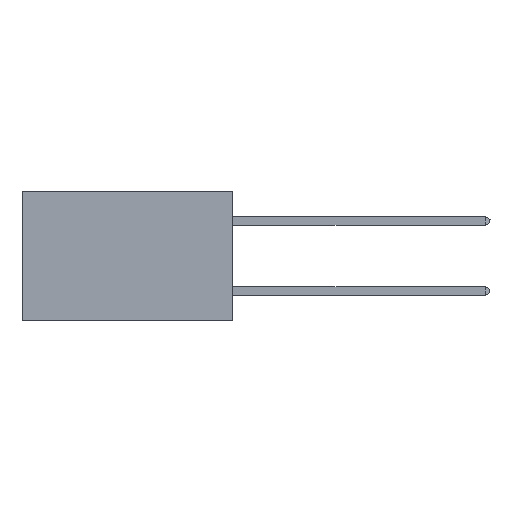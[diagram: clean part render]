
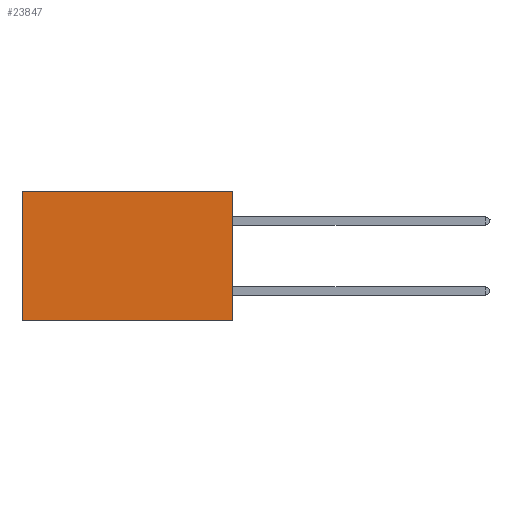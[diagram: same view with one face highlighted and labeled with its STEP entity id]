
A CAD part, left-side view. The second image highlights one B-rep face of the part: STEP entity #23847.
In plain terms, the highlighted planar face has unit normal (-1, 0, 0).
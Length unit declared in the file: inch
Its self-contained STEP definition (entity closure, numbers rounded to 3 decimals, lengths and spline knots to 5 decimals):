
#1172 = AXIS2_PLACEMENT_3D ( 'NONE', #16849, #28862, #4880 ) ;
#2089 = DIRECTION ( 'NONE',  ( 0., 1., 0. ) ) ;
#2196 = EDGE_CURVE ( 'NONE', #14320, #7238, #22679, .T. ) ;
#2697 = CARTESIAN_POINT ( 'NONE',  ( 0.2875, 0., -0.37 ) ) ;
#3125 = EDGE_CURVE ( 'NONE', #24840, #14320, #20857, .T. ) ;
#3330 = ORIENTED_EDGE ( 'NONE', *, *, #3125, .F. ) ;
#4679 = LINE ( 'NONE', #24192, #26167 ) ;
#4880 = DIRECTION ( 'NONE',  ( 0., 0., -1. ) ) ;
#6557 = VECTOR ( 'NONE', #21942, 39.37008 ) ;
#7205 = PLANE ( 'NONE',  #1172 ) ;
#7238 = VERTEX_POINT ( 'NONE', #16813 ) ;
#10974 = EDGE_CURVE ( 'NONE', #24840, #16836, #4679, .T. ) ;
#11764 = VECTOR ( 'NONE', #19516, 39.37008 ) ;
#12336 = CARTESIAN_POINT ( 'NONE',  ( 0.2875, 0., 0. ) ) ;
#12496 = EDGE_LOOP ( 'NONE', ( #23411, #29990, #3330, #21743 ) ) ;
#14320 = VERTEX_POINT ( 'NONE', #20056 ) ;
#16331 = FACE_OUTER_BOUND ( 'NONE', #12496, .T. ) ;
#16484 = CARTESIAN_POINT ( 'NONE',  ( 0.2875, 0.6, 0. ) ) ;
#16813 = CARTESIAN_POINT ( 'NONE',  ( 0.2875, 0.6, -0.37 ) ) ;
#16836 = VERTEX_POINT ( 'NONE', #26456 ) ;
#16849 = CARTESIAN_POINT ( 'NONE',  ( 0.2875, 0., 0. ) ) ;
#17337 = EDGE_CURVE ( 'NONE', #16836, #7238, #23730, .T. ) ;
#19516 = DIRECTION ( 'NONE',  ( 0., 1., 0. ) ) ;
#20056 = CARTESIAN_POINT ( 'NONE',  ( 0.2875, 0., -0.37 ) ) ;
#20857 = LINE ( 'NONE', #12336, #6557 ) ;
#21253 = DIRECTION ( 'NONE',  ( 0., 0., -1. ) ) ;
#21743 = ORIENTED_EDGE ( 'NONE', *, *, #10974, .T. ) ;
#21942 = DIRECTION ( 'NONE',  ( 0., 0., -1. ) ) ;
#22606 = VECTOR ( 'NONE', #21253, 39.37008 ) ;
#22679 = LINE ( 'NONE', #2697, #11764 ) ;
#23411 = ORIENTED_EDGE ( 'NONE', *, *, #17337, .T. ) ;
#23498 = CARTESIAN_POINT ( 'NONE',  ( 0.2875, 0., 0. ) ) ;
#23730 = LINE ( 'NONE', #16484, #22606 ) ;
#23847 = ADVANCED_FACE ( 'NONE', ( #16331 ), #7205, .F. ) ;
#24192 = CARTESIAN_POINT ( 'NONE',  ( 0.2875, 0., 0. ) ) ;
#24840 = VERTEX_POINT ( 'NONE', #23498 ) ;
#26167 = VECTOR ( 'NONE', #2089, 39.37008 ) ;
#26456 = CARTESIAN_POINT ( 'NONE',  ( 0.2875, 0.6, 0. ) ) ;
#28862 = DIRECTION ( 'NONE',  ( 1., 0., 0. ) ) ;
#29990 = ORIENTED_EDGE ( 'NONE', *, *, #2196, .F. ) ;
